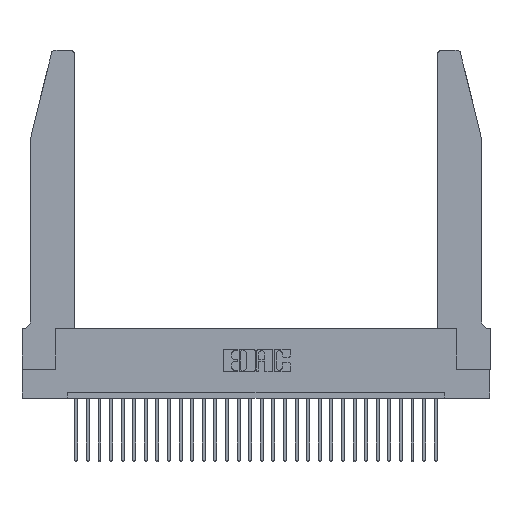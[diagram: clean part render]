
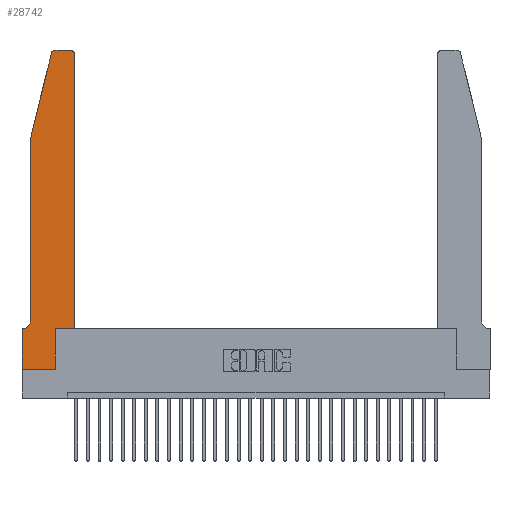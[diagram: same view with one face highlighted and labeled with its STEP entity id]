
A CAD part, top view. The second image highlights one B-rep face of the part: STEP entity #28742.
In plain terms, the highlighted planar face has unit normal (0, 0, 1).
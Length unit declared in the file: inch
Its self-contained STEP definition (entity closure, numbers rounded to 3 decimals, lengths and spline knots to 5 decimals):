
#1 = DIRECTION ( 'NONE',  ( 1., 0., 0. ) ) ;
#168 = VECTOR ( 'NONE', #1, 39.37008 ) ;
#347 = CARTESIAN_POINT ( 'NONE',  ( 0., 0.35, 0.37 ) ) ;
#501 = ORIENTED_EDGE ( 'NONE', *, *, #27430, .T. ) ;
#1132 = AXIS2_PLACEMENT_3D ( 'NONE', #6234, #20052, #10820 ) ;
#1247 = LINE ( 'NONE', #7003, #25613 ) ;
#1293 = VERTEX_POINT ( 'NONE', #11875 ) ;
#1403 = DIRECTION ( 'NONE',  ( -1., 0., 0. ) ) ;
#1671 = AXIS2_PLACEMENT_3D ( 'NONE', #22875, #17979, #15989 ) ;
#1962 = VECTOR ( 'NONE', #19888, 39.37008 ) ;
#2167 = AXIS2_PLACEMENT_3D ( 'NONE', #22513, #3942, #1403 ) ;
#2628 = LINE ( 'NONE', #22751, #8819 ) ;
#2654 = CARTESIAN_POINT ( 'NONE',  ( 0., 0., 0.37 ) ) ;
#2924 = EDGE_CURVE ( 'NONE', #8147, #3226, #9823, .T. ) ;
#3226 = VERTEX_POINT ( 'NONE', #7596 ) ;
#3536 = CIRCLE ( 'NONE', #2167, 0.07 ) ;
#3889 = ORIENTED_EDGE ( 'NONE', *, *, #20688, .T. ) ;
#3942 = DIRECTION ( 'NONE',  ( 0., 0., -1. ) ) ;
#4112 = CARTESIAN_POINT ( 'NONE',  ( 0.0755, 0.42, 0.37 ) ) ;
#4470 = DIRECTION ( 'NONE',  ( 1., 0., 0. ) ) ;
#4501 = PLANE ( 'NONE',  #1671 ) ;
#4698 = CARTESIAN_POINT ( 'NONE',  ( 0., 0., 0.37 ) ) ;
#5636 = LINE ( 'NONE', #23422, #22695 ) ;
#5712 = EDGE_CURVE ( 'NONE', #21779, #26908, #5636, .T. ) ;
#5902 = ORIENTED_EDGE ( 'NONE', *, *, #12023, .T. ) ;
#6165 = VECTOR ( 'NONE', #11074, 39.37008 ) ;
#6234 = CARTESIAN_POINT ( 'NONE',  ( 0.4205, 2.72, 0.37 ) ) ;
#7003 = CARTESIAN_POINT ( 'NONE',  ( 0.2605, 2.75, 0.37 ) ) ;
#7196 = AXIS2_PLACEMENT_3D ( 'NONE', #25619, #16158, #4470 ) ;
#7596 = CARTESIAN_POINT ( 'NONE',  ( 0.4505, 2.72, 0.37 ) ) ;
#8147 = VERTEX_POINT ( 'NONE', #10391 ) ;
#8168 = LINE ( 'NONE', #8246, #1962 ) ;
#8246 = CARTESIAN_POINT ( 'NONE',  ( 0.0755, 0.35, 0.37 ) ) ;
#8499 = FACE_OUTER_BOUND ( 'NONE', #23910, .T. ) ;
#8819 = VECTOR ( 'NONE', #9176, 39.37008 ) ;
#9176 = DIRECTION ( 'NONE',  ( 0., 1., 0. ) ) ;
#9259 = VERTEX_POINT ( 'NONE', #16244 ) ;
#9823 = LINE ( 'NONE', #29626, #6165 ) ;
#10283 = VECTOR ( 'NONE', #22565, 39.37008 ) ;
#10391 = CARTESIAN_POINT ( 'NONE',  ( 0.4505, 0.35, 0.37 ) ) ;
#10398 = LINE ( 'NONE', #4698, #168 ) ;
#10820 = DIRECTION ( 'NONE',  ( 1., 0., 0. ) ) ;
#10982 = CIRCLE ( 'NONE', #7196, 0.03 ) ;
#11074 = DIRECTION ( 'NONE',  ( 0., 1., 0. ) ) ;
#11088 = CARTESIAN_POINT ( 'NONE',  ( 0., 0., 0.37 ) ) ;
#11480 = LINE ( 'NONE', #18555, #20233 ) ;
#11875 = CARTESIAN_POINT ( 'NONE',  ( 0.0055, 0.35, 0.37 ) ) ;
#12023 = EDGE_CURVE ( 'NONE', #15417, #24630, #10982, .T. ) ;
#13075 = ORIENTED_EDGE ( 'NONE', *, *, #23321, .T. ) ;
#13427 = CARTESIAN_POINT ( 'NONE',  ( 0.4205, 2.75, 0.37 ) ) ;
#13668 = VECTOR ( 'NONE', #25339, 39.37008 ) ;
#13844 = ORIENTED_EDGE ( 'NONE', *, *, #18675, .T. ) ;
#13999 = DIRECTION ( 'NONE',  ( 0., -1., 0. ) ) ;
#14053 = LINE ( 'NONE', #11088, #13668 ) ;
#14292 = EDGE_CURVE ( 'NONE', #26908, #1293, #3536, .T. ) ;
#14590 = ORIENTED_EDGE ( 'NONE', *, *, #14292, .T. ) ;
#15384 = CARTESIAN_POINT ( 'NONE',  ( 0.0755, 2., 0.37 ) ) ;
#15417 = VERTEX_POINT ( 'NONE', #24043 ) ;
#15902 = ORIENTED_EDGE ( 'NONE', *, *, #5712, .T. ) ;
#15977 = EDGE_CURVE ( 'NONE', #1293, #30173, #8168, .T. ) ;
#15989 = DIRECTION ( 'NONE',  ( 1., 0., 0. ) ) ;
#16067 = VERTEX_POINT ( 'NONE', #13427 ) ;
#16157 = DIRECTION ( 'NONE',  ( -1., 0., 0. ) ) ;
#16158 = DIRECTION ( 'NONE',  ( 0., 0., 1. ) ) ;
#16244 = CARTESIAN_POINT ( 'NONE',  ( 0.2865, 0.35, 0.37 ) ) ;
#16704 = EDGE_CURVE ( 'NONE', #26958, #9259, #2628, .T. ) ;
#17979 = DIRECTION ( 'NONE',  ( 0., 0., 1. ) ) ;
#18461 = DIRECTION ( 'NONE',  ( 1., 0., 0. ) ) ;
#18555 = CARTESIAN_POINT ( 'NONE',  ( 0.4505, 0.35, 0.37 ) ) ;
#18675 = EDGE_CURVE ( 'NONE', #9259, #8147, #11480, .T. ) ;
#19840 = ORIENTED_EDGE ( 'NONE', *, *, #15977, .T. ) ;
#19888 = DIRECTION ( 'NONE',  ( -1., 0., 0. ) ) ;
#20052 = DIRECTION ( 'NONE',  ( 0., 0., 1. ) ) ;
#20233 = VECTOR ( 'NONE', #18461, 39.37008 ) ;
#20459 = EDGE_CURVE ( 'NONE', #30173, #25748, #14053, .T. ) ;
#20688 = EDGE_CURVE ( 'NONE', #25748, #26958, #10398, .T. ) ;
#20982 = ORIENTED_EDGE ( 'NONE', *, *, #2924, .T. ) ;
#21212 = ORIENTED_EDGE ( 'NONE', *, *, #28614, .T. ) ;
#21779 = VERTEX_POINT ( 'NONE', #26042 ) ;
#22270 = CIRCLE ( 'NONE', #1132, 0.03 ) ;
#22513 = CARTESIAN_POINT ( 'NONE',  ( 0.0055, 0.42, 0.37 ) ) ;
#22565 = DIRECTION ( 'NONE',  ( -0.239, -0.971, 0. ) ) ;
#22695 = VECTOR ( 'NONE', #13999, 39.37008 ) ;
#22751 = CARTESIAN_POINT ( 'NONE',  ( 0.2865, 0.35, 0.37 ) ) ;
#22875 = CARTESIAN_POINT ( 'NONE',  ( 0., 0.35, 0.37 ) ) ;
#23076 = ORIENTED_EDGE ( 'NONE', *, *, #16704, .T. ) ;
#23321 = EDGE_CURVE ( 'NONE', #3226, #16067, #22270, .T. ) ;
#23422 = CARTESIAN_POINT ( 'NONE',  ( 0.0755, 2., 0.37 ) ) ;
#23743 = CARTESIAN_POINT ( 'NONE',  ( 0.25487, 2.72718, 0.37 ) ) ;
#23910 = EDGE_LOOP ( 'NONE', ( #501, #5902, #21212, #15902, #14590, #19840, #29276, #3889, #23076, #13844, #20982, #13075 ) ) ;
#24043 = CARTESIAN_POINT ( 'NONE',  ( 0.284, 2.75, 0.37 ) ) ;
#24630 = VERTEX_POINT ( 'NONE', #23743 ) ;
#24753 = CARTESIAN_POINT ( 'NONE',  ( 0.2865, 0., 0.37 ) ) ;
#25339 = DIRECTION ( 'NONE',  ( 0., -1., 0. ) ) ;
#25613 = VECTOR ( 'NONE', #16157, 39.37008 ) ;
#25619 = CARTESIAN_POINT ( 'NONE',  ( 0.284, 2.72, 0.37 ) ) ;
#25748 = VERTEX_POINT ( 'NONE', #2654 ) ;
#26042 = CARTESIAN_POINT ( 'NONE',  ( 0.0755, 2., 0.37 ) ) ;
#26908 = VERTEX_POINT ( 'NONE', #4112 ) ;
#26958 = VERTEX_POINT ( 'NONE', #24753 ) ;
#27076 = LINE ( 'NONE', #15384, #10283 ) ;
#27430 = EDGE_CURVE ( 'NONE', #16067, #15417, #1247, .T. ) ;
#28614 = EDGE_CURVE ( 'NONE', #24630, #21779, #27076, .T. ) ;
#28742 = ADVANCED_FACE ( 'NONE', ( #8499 ), #4501, .T. ) ;
#29276 = ORIENTED_EDGE ( 'NONE', *, *, #20459, .T. ) ;
#29626 = CARTESIAN_POINT ( 'NONE',  ( 0.4505, 0.35, 0.37 ) ) ;
#30173 = VERTEX_POINT ( 'NONE', #347 ) ;
